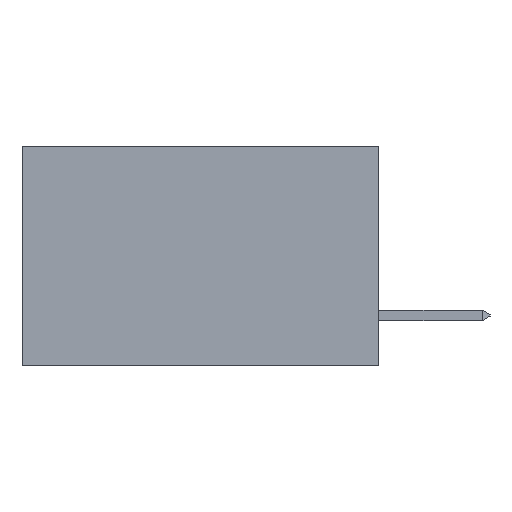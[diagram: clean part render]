
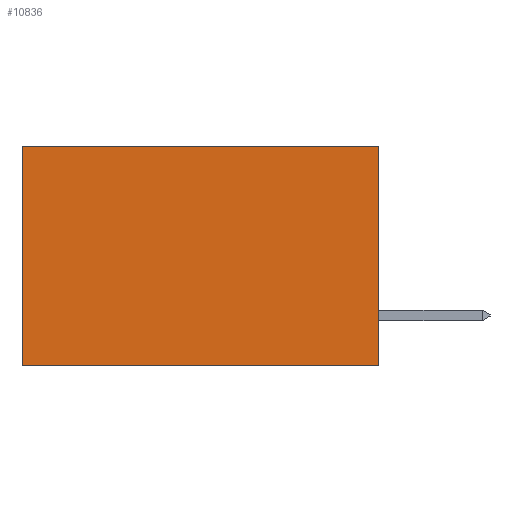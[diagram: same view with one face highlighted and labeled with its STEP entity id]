
A CAD part, left-side view. The second image highlights one B-rep face of the part: STEP entity #10836.
In plain terms, the highlighted planar face has unit normal (-1, 0, 0).
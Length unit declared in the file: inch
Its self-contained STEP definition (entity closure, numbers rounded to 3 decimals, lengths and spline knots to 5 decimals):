
#286 = EDGE_CURVE ( 'NONE', #1574, #11072, #10252, .T. ) ;
#1045 = ORIENTED_EDGE ( 'NONE', *, *, #286, .T. ) ;
#1574 = VERTEX_POINT ( 'NONE', #2492 ) ;
#1721 = CARTESIAN_POINT ( 'NONE',  ( 0.298, 0.6, 0. ) ) ;
#2135 = CARTESIAN_POINT ( 'NONE',  ( 0.298, 0., -0.37 ) ) ;
#2386 = ORIENTED_EDGE ( 'NONE', *, *, #4288, .F. ) ;
#2492 = CARTESIAN_POINT ( 'NONE',  ( 0.298, 0., 0. ) ) ;
#2553 = AXIS2_PLACEMENT_3D ( 'NONE', #9534, #9094, #9001 ) ;
#2789 = EDGE_CURVE ( 'NONE', #11072, #3226, #6497, .T. ) ;
#2969 = EDGE_LOOP ( 'NONE', ( #8745, #10537, #2386, #1045 ) ) ;
#3068 = VERTEX_POINT ( 'NONE', #2135 ) ;
#3226 = VERTEX_POINT ( 'NONE', #10163 ) ;
#3911 = DIRECTION ( 'NONE',  ( 0., 1., 0. ) ) ;
#4032 = VECTOR ( 'NONE', #4152, 39.37008 ) ;
#4071 = CARTESIAN_POINT ( 'NONE',  ( 0.298, 0.6, 0. ) ) ;
#4152 = DIRECTION ( 'NONE',  ( 0., 0., -1. ) ) ;
#4288 = EDGE_CURVE ( 'NONE', #1574, #3068, #10006, .T. ) ;
#5025 = DIRECTION ( 'NONE',  ( 0., 0., -1. ) ) ;
#6497 = LINE ( 'NONE', #4071, #4032 ) ;
#6845 = CARTESIAN_POINT ( 'NONE',  ( 0.298, 0., 0. ) ) ;
#7158 = VECTOR ( 'NONE', #11850, 39.37008 ) ;
#7424 = LINE ( 'NONE', #11713, #7158 ) ;
#7949 = VECTOR ( 'NONE', #3911, 39.37008 ) ;
#8227 = CARTESIAN_POINT ( 'NONE',  ( 0.298, 0., 0. ) ) ;
#8537 = EDGE_CURVE ( 'NONE', #3068, #3226, #7424, .T. ) ;
#8745 = ORIENTED_EDGE ( 'NONE', *, *, #2789, .T. ) ;
#8885 = FACE_OUTER_BOUND ( 'NONE', #2969, .T. ) ;
#9001 = DIRECTION ( 'NONE',  ( 0., 0., -1. ) ) ;
#9094 = DIRECTION ( 'NONE',  ( 1., 0., 0. ) ) ;
#9430 = PLANE ( 'NONE',  #2553 ) ;
#9534 = CARTESIAN_POINT ( 'NONE',  ( 0.298, 0., 0. ) ) ;
#10006 = LINE ( 'NONE', #8227, #11989 ) ;
#10163 = CARTESIAN_POINT ( 'NONE',  ( 0.298, 0.6, -0.37 ) ) ;
#10252 = LINE ( 'NONE', #6845, #7949 ) ;
#10537 = ORIENTED_EDGE ( 'NONE', *, *, #8537, .F. ) ;
#10836 = ADVANCED_FACE ( 'NONE', ( #8885 ), #9430, .F. ) ;
#11072 = VERTEX_POINT ( 'NONE', #1721 ) ;
#11713 = CARTESIAN_POINT ( 'NONE',  ( 0.298, 0., -0.37 ) ) ;
#11850 = DIRECTION ( 'NONE',  ( 0., 1., 0. ) ) ;
#11989 = VECTOR ( 'NONE', #5025, 39.37008 ) ;
